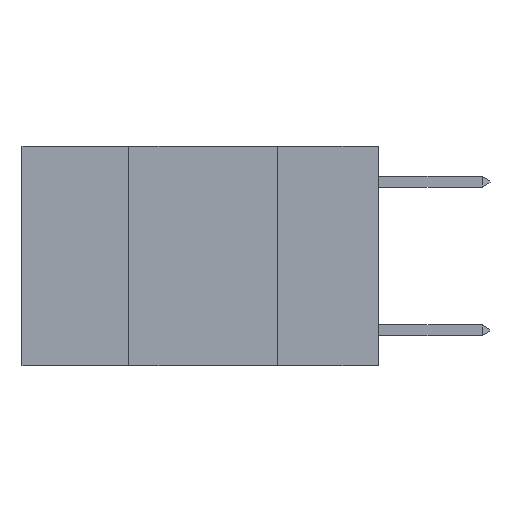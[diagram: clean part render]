
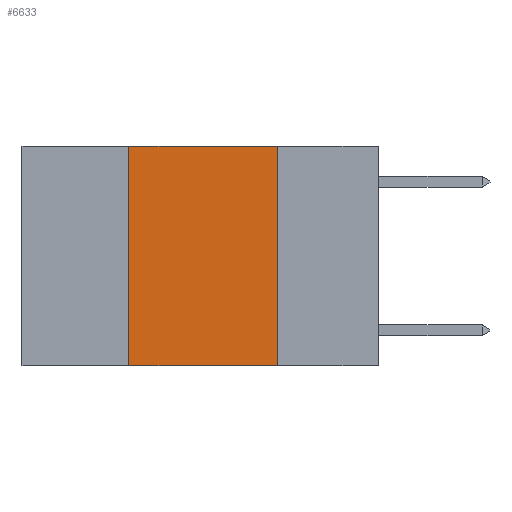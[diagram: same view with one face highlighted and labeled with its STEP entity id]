
A CAD part, left-side view. The second image highlights one B-rep face of the part: STEP entity #6633.
In plain terms, the highlighted planar face has unit normal (-1, 0, 0).
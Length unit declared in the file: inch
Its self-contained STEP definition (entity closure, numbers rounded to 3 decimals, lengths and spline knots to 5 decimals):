
#38 = AXIS2_PLACEMENT_3D ( 'NONE', #1664, #8021, #2600 ) ;
#129 = VERTEX_POINT ( 'NONE', #6686 ) ;
#166 = FACE_OUTER_BOUND ( 'NONE', #4166, .T. ) ;
#420 = CARTESIAN_POINT ( 'NONE',  ( 0., 0.6, 0. ) ) ;
#913 = EDGE_CURVE ( 'NONE', #7317, #129, #10968, .T. ) ;
#1664 = CARTESIAN_POINT ( 'NONE',  ( 0., 0.6, 0. ) ) ;
#1798 = VECTOR ( 'NONE', #5152, 39.37008 ) ;
#2364 = CARTESIAN_POINT ( 'NONE',  ( 0., 0.42, 0. ) ) ;
#2600 = DIRECTION ( 'NONE',  ( 0., 0., -1. ) ) ;
#3865 = VECTOR ( 'NONE', #10336, 39.37008 ) ;
#3974 = LINE ( 'NONE', #420, #1798 ) ;
#3997 = CARTESIAN_POINT ( 'NONE',  ( 0., 0.17, 0. ) ) ;
#4166 = EDGE_LOOP ( 'NONE', ( #7454, #7392, #6445, #6174 ) ) ;
#4589 = LINE ( 'NONE', #6899, #11369 ) ;
#5152 = DIRECTION ( 'NONE',  ( 0., -1., 0. ) ) ;
#6174 = ORIENTED_EDGE ( 'NONE', *, *, #10966, .T. ) ;
#6445 = ORIENTED_EDGE ( 'NONE', *, *, #6476, .F. ) ;
#6476 = EDGE_CURVE ( 'NONE', #7548, #8415, #9231, .T. ) ;
#6633 = ADVANCED_FACE ( 'NONE', ( #166 ), #11520, .F. ) ;
#6686 = CARTESIAN_POINT ( 'NONE',  ( 0., 0.17, -0.37 ) ) ;
#6881 = DIRECTION ( 'NONE',  ( 0., 0., 1. ) ) ;
#6899 = CARTESIAN_POINT ( 'NONE',  ( 0., 0.6, -0.37 ) ) ;
#7317 = VERTEX_POINT ( 'NONE', #3997 ) ;
#7392 = ORIENTED_EDGE ( 'NONE', *, *, #9449, .F. ) ;
#7454 = ORIENTED_EDGE ( 'NONE', *, *, #913, .F. ) ;
#7548 = VERTEX_POINT ( 'NONE', #11364 ) ;
#8021 = DIRECTION ( 'NONE',  ( 1., 0., 0. ) ) ;
#8095 = CARTESIAN_POINT ( 'NONE',  ( 0., 0.42, 0. ) ) ;
#8415 = VERTEX_POINT ( 'NONE', #8095 ) ;
#8704 = DIRECTION ( 'NONE',  ( 0., -1., 0. ) ) ;
#9231 = LINE ( 'NONE', #2364, #11266 ) ;
#9449 = EDGE_CURVE ( 'NONE', #8415, #7317, #3974, .T. ) ;
#9460 = CARTESIAN_POINT ( 'NONE',  ( 0., 0.17, 0. ) ) ;
#10336 = DIRECTION ( 'NONE',  ( 0., 0., -1. ) ) ;
#10966 = EDGE_CURVE ( 'NONE', #7548, #129, #4589, .T. ) ;
#10968 = LINE ( 'NONE', #9460, #3865 ) ;
#11266 = VECTOR ( 'NONE', #6881, 39.37008 ) ;
#11364 = CARTESIAN_POINT ( 'NONE',  ( 0., 0.42, -0.37 ) ) ;
#11369 = VECTOR ( 'NONE', #8704, 39.37008 ) ;
#11520 = PLANE ( 'NONE',  #38 ) ;
